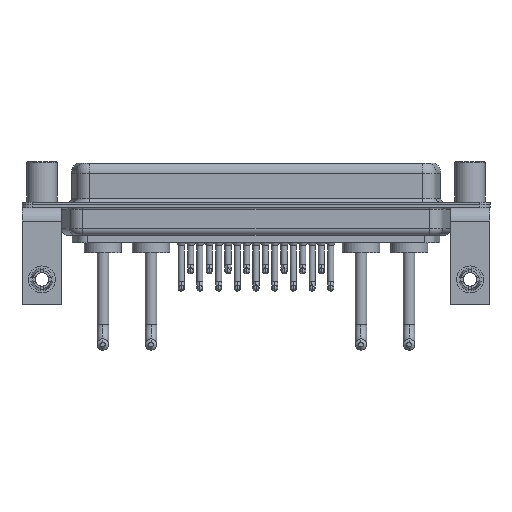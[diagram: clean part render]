
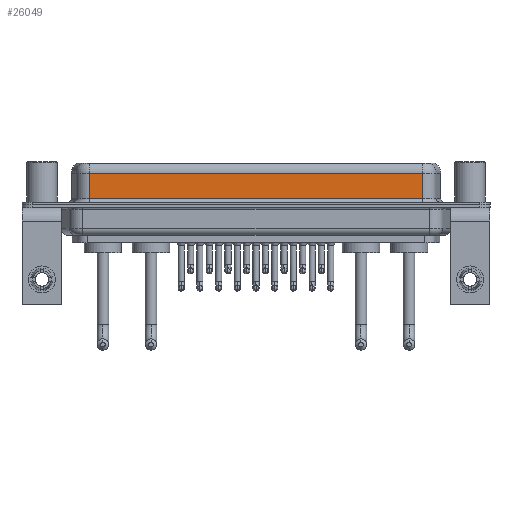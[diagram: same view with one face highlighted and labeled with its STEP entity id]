
A CAD part, front view. The second image highlights one B-rep face of the part: STEP entity #26049.
In plain terms, the highlighted planar face has unit normal (0, -1, 0).
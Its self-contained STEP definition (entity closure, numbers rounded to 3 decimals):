
#78 = CARTESIAN_POINT ( 'NONE',  ( 56.462, -3.95, 4.65 ) ) ;
#139 = EDGE_CURVE ( 'NONE', #2966, #23114, #7652, .T. ) ;
#1044 = VECTOR ( 'NONE', #25576, 1000. ) ;
#1336 = CARTESIAN_POINT ( 'NONE',  ( 56.462, -3.95, 0.9 ) ) ;
#1437 = AXIS2_PLACEMENT_3D ( 'NONE', #22967, #10785, #11298 ) ;
#2966 = VERTEX_POINT ( 'NONE', #78 ) ;
#3234 = FACE_OUTER_BOUND ( 'NONE', #10685, .T. ) ;
#3866 = CARTESIAN_POINT ( 'NONE',  ( 7.038, -3.95, 4.65 ) ) ;
#4862 = EDGE_CURVE ( 'NONE', #23114, #7375, #18519, .T. ) ;
#4929 = CARTESIAN_POINT ( 'NONE',  ( 56.462, -3.95, 6.4 ) ) ;
#5058 = VERTEX_POINT ( 'NONE', #8854 ) ;
#5158 = ORIENTED_EDGE ( 'NONE', *, *, #25172, .T. ) ;
#6514 = ORIENTED_EDGE ( 'NONE', *, *, #139, .T. ) ;
#6657 = LINE ( 'NONE', #4929, #12184 ) ;
#7130 = DIRECTION ( 'NONE',  ( -1., 0., 0. ) ) ;
#7375 = VERTEX_POINT ( 'NONE', #10900 ) ;
#7652 = LINE ( 'NONE', #9366, #21959 ) ;
#7748 = VECTOR ( 'NONE', #10164, 1000. ) ;
#8854 = CARTESIAN_POINT ( 'NONE',  ( 56.462, -3.95, 0.9 ) ) ;
#9366 = CARTESIAN_POINT ( 'NONE',  ( 56.462, -3.95, 4.65 ) ) ;
#10164 = DIRECTION ( 'NONE',  ( 0., 0., -1. ) ) ;
#10184 = ORIENTED_EDGE ( 'NONE', *, *, #4862, .T. ) ;
#10685 = EDGE_LOOP ( 'NONE', ( #13736, #6514, #10184, #5158 ) ) ;
#10785 = DIRECTION ( 'NONE',  ( 0., 1., 0. ) ) ;
#10900 = CARTESIAN_POINT ( 'NONE',  ( 7.038, -3.95, 0.9 ) ) ;
#11034 = PLANE ( 'NONE',  #1437 ) ;
#11298 = DIRECTION ( 'NONE',  ( 0., 0., 1. ) ) ;
#12184 = VECTOR ( 'NONE', #25050, 1000. ) ;
#12269 = EDGE_CURVE ( 'NONE', #2966, #5058, #6657, .T. ) ;
#13736 = ORIENTED_EDGE ( 'NONE', *, *, #12269, .F. ) ;
#18519 = LINE ( 'NONE', #20241, #7748 ) ;
#19473 = LINE ( 'NONE', #1336, #1044 ) ;
#20241 = CARTESIAN_POINT ( 'NONE',  ( 7.038, -3.95, 6.4 ) ) ;
#21959 = VECTOR ( 'NONE', #7130, 1000. ) ;
#22967 = CARTESIAN_POINT ( 'NONE',  ( 56.462, -3.95, 6.4 ) ) ;
#23114 = VERTEX_POINT ( 'NONE', #3866 ) ;
#25050 = DIRECTION ( 'NONE',  ( 0., 0., -1. ) ) ;
#25172 = EDGE_CURVE ( 'NONE', #7375, #5058, #19473, .T. ) ;
#25576 = DIRECTION ( 'NONE',  ( 1., 0., 0. ) ) ;
#26049 = ADVANCED_FACE ( 'NONE', ( #3234 ), #11034, .F. ) ;
